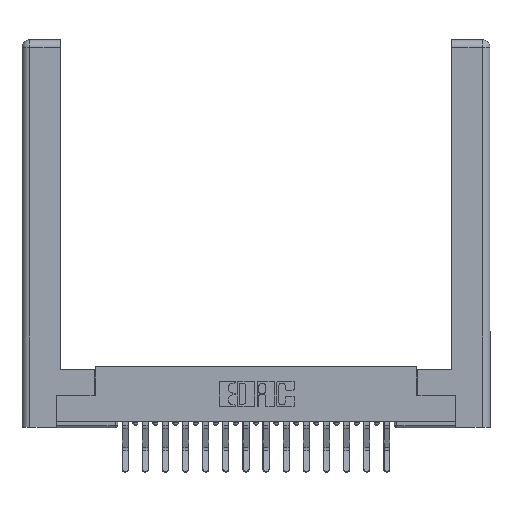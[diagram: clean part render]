
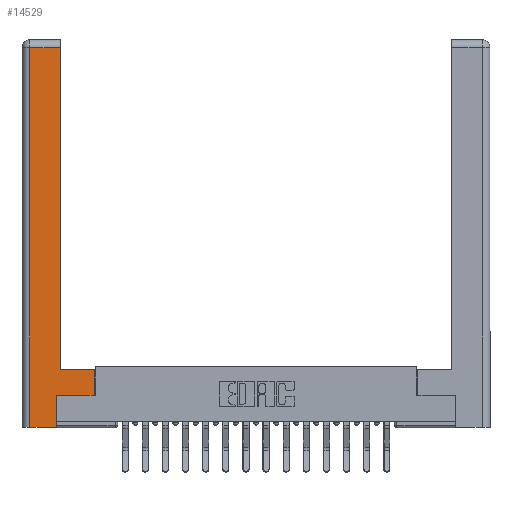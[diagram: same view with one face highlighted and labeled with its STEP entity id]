
A CAD part, top view. The second image highlights one B-rep face of the part: STEP entity #14529.
In plain terms, the highlighted planar face has unit normal (0, 0, 1).
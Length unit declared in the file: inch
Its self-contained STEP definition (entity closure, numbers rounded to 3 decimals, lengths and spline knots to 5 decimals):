
#254 = EDGE_CURVE ( 'NONE', #2796, #10131, #5986, .T. ) ;
#392 = CARTESIAN_POINT ( 'NONE',  ( 0.265, 0., 0. ) ) ;
#627 = DIRECTION ( 'NONE',  ( 0., 1., 0. ) ) ;
#812 = CARTESIAN_POINT ( 'NONE',  ( 0.565, 0.245, 0. ) ) ;
#1364 = ORIENTED_EDGE ( 'NONE', *, *, #1901, .T. ) ;
#1424 = DIRECTION ( 'NONE',  ( -1., 0., 0. ) ) ;
#1756 = CARTESIAN_POINT ( 'NONE',  ( 0.0615, 0., 0. ) ) ;
#1901 = EDGE_CURVE ( 'NONE', #15971, #8480, #17370, .T. ) ;
#2416 = DIRECTION ( 'NONE',  ( 1., 0., 0. ) ) ;
#2796 = VERTEX_POINT ( 'NONE', #9229 ) ;
#3115 = VECTOR ( 'NONE', #627, 39.37008 ) ;
#3447 = CARTESIAN_POINT ( 'NONE',  ( 0.0615, 2.94, 0. ) ) ;
#3721 = DIRECTION ( 'NONE',  ( 0., 1., 0. ) ) ;
#4663 = EDGE_CURVE ( 'NONE', #10131, #12818, #15686, .T. ) ;
#4800 = EDGE_CURVE ( 'NONE', #12818, #17578, #14731, .T. ) ;
#5336 = EDGE_CURVE ( 'NONE', #15900, #18654, #13744, .T. ) ;
#5809 = VECTOR ( 'NONE', #2416, 39.37008 ) ;
#5818 = CARTESIAN_POINT ( 'NONE',  ( 0.295, 0.45, 0. ) ) ;
#5865 = CARTESIAN_POINT ( 'NONE',  ( 0.565, 0.245, 0. ) ) ;
#5883 = CARTESIAN_POINT ( 'NONE',  ( 0.295, 0.45, 0. ) ) ;
#5986 = LINE ( 'NONE', #3447, #10838 ) ;
#6168 = EDGE_CURVE ( 'NONE', #18654, #15971, #17948, .T. ) ;
#6180 = DIRECTION ( 'NONE',  ( 1., 0., 0. ) ) ;
#6526 = ORIENTED_EDGE ( 'NONE', *, *, #5336, .T. ) ;
#6744 = VECTOR ( 'NONE', #3721, 39.37008 ) ;
#7137 = CARTESIAN_POINT ( 'NONE',  ( 0.265, 0., 0. ) ) ;
#7238 = CARTESIAN_POINT ( 'NONE',  ( 0., 0., 0. ) ) ;
#7304 = CARTESIAN_POINT ( 'NONE',  ( 0.0615, 0., 0. ) ) ;
#7546 = CARTESIAN_POINT ( 'NONE',  ( 0.265, 0.245, 0. ) ) ;
#7776 = DIRECTION ( 'NONE',  ( 0., 1., 0. ) ) ;
#7867 = CARTESIAN_POINT ( 'NONE',  ( 0.295, 3., 0. ) ) ;
#8128 = EDGE_LOOP ( 'NONE', ( #13936, #14030, #8913, #12375, #9998, #6526, #13522, #1364 ) ) ;
#8480 = VERTEX_POINT ( 'NONE', #5818 ) ;
#8531 = DIRECTION ( 'NONE',  ( 0., -1., 0. ) ) ;
#8568 = PLANE ( 'NONE',  #16942 ) ;
#8913 = ORIENTED_EDGE ( 'NONE', *, *, #4663, .T. ) ;
#9099 = VECTOR ( 'NONE', #8531, 39.37008 ) ;
#9153 = LINE ( 'NONE', #7546, #3115 ) ;
#9223 = CARTESIAN_POINT ( 'NONE',  ( 0.265, 0.245, 0. ) ) ;
#9229 = CARTESIAN_POINT ( 'NONE',  ( 0.295, 2.94, 0. ) ) ;
#9400 = VECTOR ( 'NONE', #6180, 39.37008 ) ;
#9977 = FACE_OUTER_BOUND ( 'NONE', #8128, .T. ) ;
#9998 = ORIENTED_EDGE ( 'NONE', *, *, #15363, .T. ) ;
#10131 = VERTEX_POINT ( 'NONE', #13810 ) ;
#10498 = LINE ( 'NONE', #7867, #12743 ) ;
#10838 = VECTOR ( 'NONE', #12097, 39.37008 ) ;
#10872 = CARTESIAN_POINT ( 'NONE',  ( 0.565, 0.45, 0. ) ) ;
#11575 = DIRECTION ( 'NONE',  ( 0., 0., -1. ) ) ;
#11967 = EDGE_CURVE ( 'NONE', #8480, #2796, #10498, .T. ) ;
#12097 = DIRECTION ( 'NONE',  ( -1., 0., 0. ) ) ;
#12375 = ORIENTED_EDGE ( 'NONE', *, *, #4800, .T. ) ;
#12625 = VECTOR ( 'NONE', #1424, 39.37008 ) ;
#12743 = VECTOR ( 'NONE', #7776, 39.37008 ) ;
#12818 = VERTEX_POINT ( 'NONE', #1756 ) ;
#12883 = DIRECTION ( 'NONE',  ( -1., 0., 0. ) ) ;
#13522 = ORIENTED_EDGE ( 'NONE', *, *, #6168, .T. ) ;
#13744 = LINE ( 'NONE', #812, #5809 ) ;
#13810 = CARTESIAN_POINT ( 'NONE',  ( 0.0615, 2.94, 0. ) ) ;
#13936 = ORIENTED_EDGE ( 'NONE', *, *, #11967, .T. ) ;
#14030 = ORIENTED_EDGE ( 'NONE', *, *, #254, .T. ) ;
#14529 = ADVANCED_FACE ( 'NONE', ( #9977 ), #8568, .F. ) ;
#14731 = LINE ( 'NONE', #392, #9400 ) ;
#15363 = EDGE_CURVE ( 'NONE', #17578, #15900, #9153, .T. ) ;
#15686 = LINE ( 'NONE', #7304, #9099 ) ;
#15900 = VERTEX_POINT ( 'NONE', #9223 ) ;
#15971 = VERTEX_POINT ( 'NONE', #16463 ) ;
#16463 = CARTESIAN_POINT ( 'NONE',  ( 0.565, 0.45, 0. ) ) ;
#16942 = AXIS2_PLACEMENT_3D ( 'NONE', #7238, #11575, #12883 ) ;
#17370 = LINE ( 'NONE', #5883, #12625 ) ;
#17578 = VERTEX_POINT ( 'NONE', #7137 ) ;
#17948 = LINE ( 'NONE', #10872, #6744 ) ;
#18654 = VERTEX_POINT ( 'NONE', #5865 ) ;
